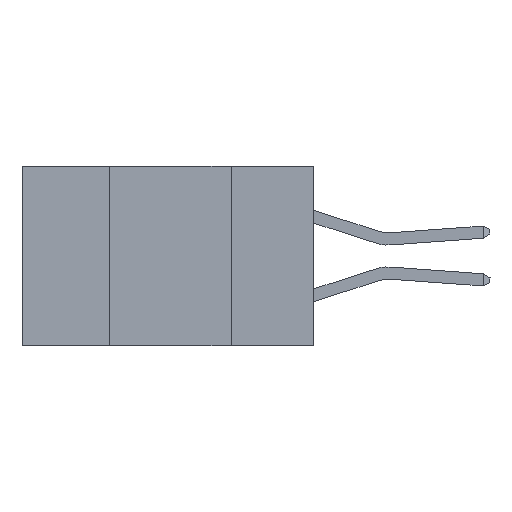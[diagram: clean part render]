
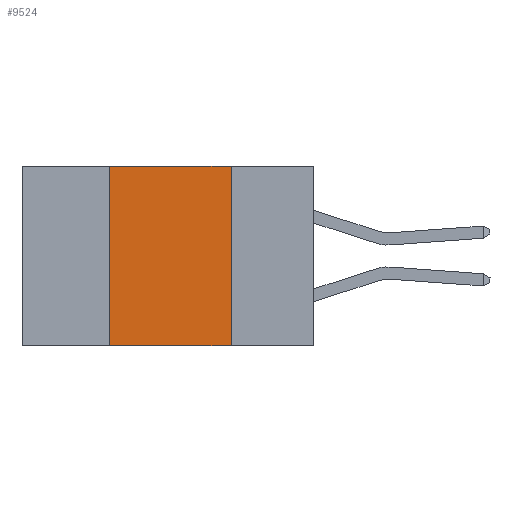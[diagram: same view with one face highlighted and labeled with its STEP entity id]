
A CAD part, left-side view. The second image highlights one B-rep face of the part: STEP entity #9524.
In plain terms, the highlighted planar face has unit normal (-1, 0, 0).
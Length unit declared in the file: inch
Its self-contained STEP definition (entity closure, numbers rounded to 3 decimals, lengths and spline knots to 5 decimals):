
#285 = DIRECTION ( 'NONE',  ( 0., 0., -1. ) ) ;
#641 = CARTESIAN_POINT ( 'NONE',  ( 0., 0.6, 0. ) ) ;
#2034 = DIRECTION ( 'NONE',  ( 0., -1., 0. ) ) ;
#2677 = VERTEX_POINT ( 'NONE', #5286 ) ;
#4615 = CARTESIAN_POINT ( 'NONE',  ( 0., 0.17, 0. ) ) ;
#4618 = FACE_OUTER_BOUND ( 'NONE', #7156, .T. ) ;
#4819 = VERTEX_POINT ( 'NONE', #7978 ) ;
#4961 = CARTESIAN_POINT ( 'NONE',  ( 0., 0.6, 0. ) ) ;
#5286 = CARTESIAN_POINT ( 'NONE',  ( 0., 0.17, -0.37 ) ) ;
#5498 = LINE ( 'NONE', #641, #14436 ) ;
#6278 = DIRECTION ( 'NONE',  ( 0., 0., -1. ) ) ;
#6380 = VECTOR ( 'NONE', #9948, 39.37008 ) ;
#7156 = EDGE_LOOP ( 'NONE', ( #15877, #7246, #8421, #15281 ) ) ;
#7246 = ORIENTED_EDGE ( 'NONE', *, *, #8186, .F. ) ;
#7978 = CARTESIAN_POINT ( 'NONE',  ( 0., 0.42, -0.37 ) ) ;
#8186 = EDGE_CURVE ( 'NONE', #11812, #12367, #5498, .T. ) ;
#8421 = ORIENTED_EDGE ( 'NONE', *, *, #11825, .F. ) ;
#9007 = LINE ( 'NONE', #15787, #9406 ) ;
#9406 = VECTOR ( 'NONE', #9514, 39.37008 ) ;
#9417 = LINE ( 'NONE', #10011, #6380 ) ;
#9514 = DIRECTION ( 'NONE',  ( 0., -1., 0. ) ) ;
#9524 = ADVANCED_FACE ( 'NONE', ( #4618 ), #11394, .F. ) ;
#9948 = DIRECTION ( 'NONE',  ( 0., 0., 1. ) ) ;
#10011 = CARTESIAN_POINT ( 'NONE',  ( 0., 0.42, 0. ) ) ;
#10651 = VECTOR ( 'NONE', #285, 39.37008 ) ;
#11394 = PLANE ( 'NONE',  #15361 ) ;
#11812 = VERTEX_POINT ( 'NONE', #16302 ) ;
#11825 = EDGE_CURVE ( 'NONE', #4819, #11812, #9417, .T. ) ;
#12367 = VERTEX_POINT ( 'NONE', #4615 ) ;
#13883 = DIRECTION ( 'NONE',  ( 1., 0., 0. ) ) ;
#14271 = EDGE_CURVE ( 'NONE', #12367, #2677, #16946, .T. ) ;
#14436 = VECTOR ( 'NONE', #2034, 39.37008 ) ;
#15281 = ORIENTED_EDGE ( 'NONE', *, *, #16195, .T. ) ;
#15361 = AXIS2_PLACEMENT_3D ( 'NONE', #4961, #13883, #6278 ) ;
#15787 = CARTESIAN_POINT ( 'NONE',  ( 0., 0.6, -0.37 ) ) ;
#15877 = ORIENTED_EDGE ( 'NONE', *, *, #14271, .F. ) ;
#15957 = CARTESIAN_POINT ( 'NONE',  ( 0., 0.17, 0. ) ) ;
#16195 = EDGE_CURVE ( 'NONE', #4819, #2677, #9007, .T. ) ;
#16302 = CARTESIAN_POINT ( 'NONE',  ( 0., 0.42, 0. ) ) ;
#16946 = LINE ( 'NONE', #15957, #10651 ) ;
